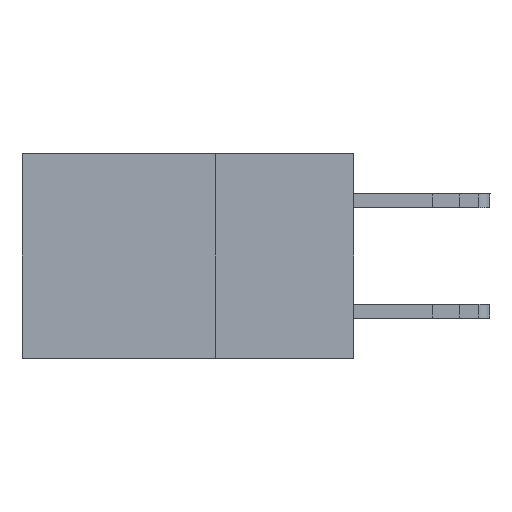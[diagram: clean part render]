
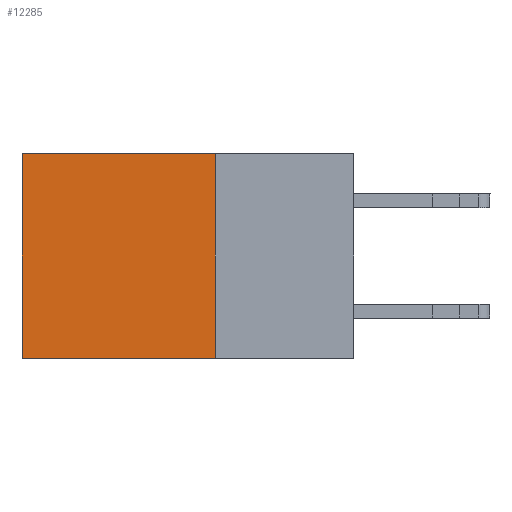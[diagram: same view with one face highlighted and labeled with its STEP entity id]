
A CAD part, left-side view. The second image highlights one B-rep face of the part: STEP entity #12285.
In plain terms, the highlighted planar face has unit normal (-1, 0, 0).
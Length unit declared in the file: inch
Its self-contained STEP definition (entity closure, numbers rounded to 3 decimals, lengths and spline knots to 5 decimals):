
#357 = AXIS2_PLACEMENT_3D ( 'NONE', #14636, #13231, #5723 ) ;
#417 = DIRECTION ( 'NONE',  ( 0., 0., -1. ) ) ;
#1429 = DIRECTION ( 'NONE',  ( 0., 1., 0. ) ) ;
#2110 = EDGE_LOOP ( 'NONE', ( #9071, #4841, #10925, #4020 ) ) ;
#2907 = DIRECTION ( 'NONE',  ( 0., 1., 0. ) ) ;
#2983 = LINE ( 'NONE', #17779, #9748 ) ;
#2997 = CARTESIAN_POINT ( 'NONE',  ( 0.2875, 0.6, -0.37 ) ) ;
#3368 = VERTEX_POINT ( 'NONE', #8073 ) ;
#4020 = ORIENTED_EDGE ( 'NONE', *, *, #6370, .T. ) ;
#4133 = LINE ( 'NONE', #5965, #6686 ) ;
#4511 = CARTESIAN_POINT ( 'NONE',  ( 0.2875, 0.6, 0. ) ) ;
#4841 = ORIENTED_EDGE ( 'NONE', *, *, #14468, .F. ) ;
#5723 = DIRECTION ( 'NONE',  ( 0., 0., -1. ) ) ;
#5965 = CARTESIAN_POINT ( 'NONE',  ( 0.2875, 0.25, -0.37 ) ) ;
#6370 = EDGE_CURVE ( 'NONE', #10443, #3368, #2983, .T. ) ;
#6405 = VERTEX_POINT ( 'NONE', #11896 ) ;
#6686 = VECTOR ( 'NONE', #1429, 39.37008 ) ;
#7176 = CARTESIAN_POINT ( 'NONE',  ( 0.2875, 0.25, 0. ) ) ;
#8073 = CARTESIAN_POINT ( 'NONE',  ( 0.2875, 0.6, 0. ) ) ;
#9026 = EDGE_CURVE ( 'NONE', #3368, #17572, #18713, .T. ) ;
#9071 = ORIENTED_EDGE ( 'NONE', *, *, #9026, .T. ) ;
#9748 = VECTOR ( 'NONE', #2907, 39.37008 ) ;
#10443 = VERTEX_POINT ( 'NONE', #7176 ) ;
#10925 = ORIENTED_EDGE ( 'NONE', *, *, #14951, .F. ) ;
#11896 = CARTESIAN_POINT ( 'NONE',  ( 0.2875, 0.25, -0.37 ) ) ;
#12285 = ADVANCED_FACE ( 'NONE', ( #14911 ), #13175, .F. ) ;
#12620 = CARTESIAN_POINT ( 'NONE',  ( 0.2875, 0.25, 0. ) ) ;
#13175 = PLANE ( 'NONE',  #357 ) ;
#13231 = DIRECTION ( 'NONE',  ( 1., 0., 0. ) ) ;
#14352 = DIRECTION ( 'NONE',  ( 0., 0., -1. ) ) ;
#14468 = EDGE_CURVE ( 'NONE', #6405, #17572, #4133, .T. ) ;
#14636 = CARTESIAN_POINT ( 'NONE',  ( 0.2875, 0.25, 0. ) ) ;
#14911 = FACE_OUTER_BOUND ( 'NONE', #2110, .T. ) ;
#14951 = EDGE_CURVE ( 'NONE', #10443, #6405, #16881, .T. ) ;
#15259 = VECTOR ( 'NONE', #14352, 39.37008 ) ;
#16585 = VECTOR ( 'NONE', #417, 39.37008 ) ;
#16881 = LINE ( 'NONE', #12620, #15259 ) ;
#17572 = VERTEX_POINT ( 'NONE', #2997 ) ;
#17779 = CARTESIAN_POINT ( 'NONE',  ( 0.2875, 0.25, 0. ) ) ;
#18713 = LINE ( 'NONE', #4511, #16585 ) ;
